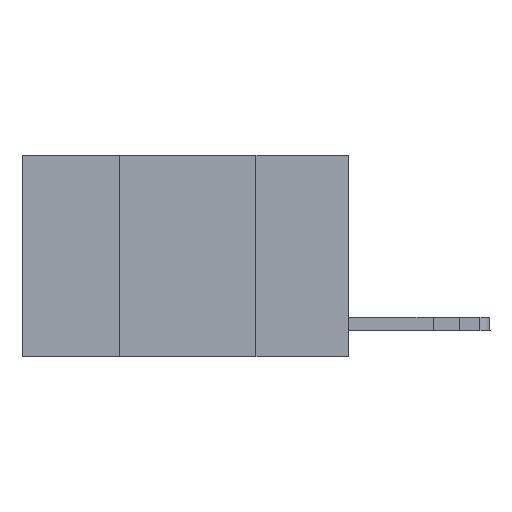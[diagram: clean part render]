
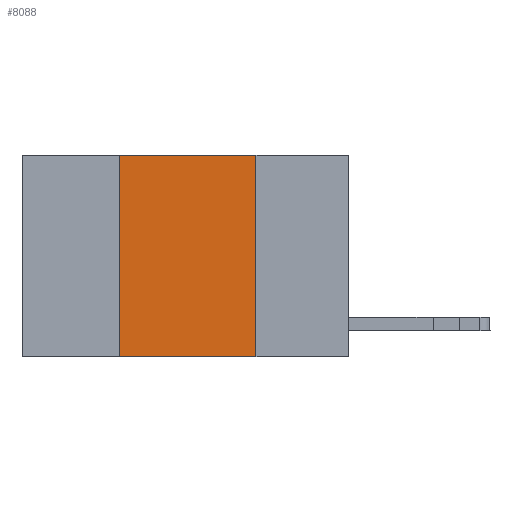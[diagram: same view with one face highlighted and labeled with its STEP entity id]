
A CAD part, left-side view. The second image highlights one B-rep face of the part: STEP entity #8088.
In plain terms, the highlighted planar face has unit normal (-1, 0, 0).
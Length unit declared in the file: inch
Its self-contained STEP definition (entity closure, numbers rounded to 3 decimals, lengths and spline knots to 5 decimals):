
#32 = CARTESIAN_POINT ( 'NONE',  ( 0., 0.17, 0. ) ) ;
#846 = LINE ( 'NONE', #9494, #6445 ) ;
#981 = DIRECTION ( 'NONE',  ( 0., 0., -1. ) ) ;
#1046 = VERTEX_POINT ( 'NONE', #12413 ) ;
#1283 = DIRECTION ( 'NONE',  ( 0., -1., 0. ) ) ;
#1828 = AXIS2_PLACEMENT_3D ( 'NONE', #13999, #7618, #981 ) ;
#1960 = DIRECTION ( 'NONE',  ( 0., 0., 1. ) ) ;
#2311 = ORIENTED_EDGE ( 'NONE', *, *, #13377, .F. ) ;
#2514 = CARTESIAN_POINT ( 'NONE',  ( 0., 0.42, -0.37 ) ) ;
#2594 = LINE ( 'NONE', #4907, #7962 ) ;
#2928 = EDGE_CURVE ( 'NONE', #7114, #14189, #13851, .T. ) ;
#3056 = DIRECTION ( 'NONE',  ( 0., 0., -1. ) ) ;
#3088 = FACE_OUTER_BOUND ( 'NONE', #8971, .T. ) ;
#4907 = CARTESIAN_POINT ( 'NONE',  ( 0., 0.6, -0.37 ) ) ;
#5120 = EDGE_CURVE ( 'NONE', #12855, #1046, #2594, .T. ) ;
#5197 = CARTESIAN_POINT ( 'NONE',  ( 0., 0.17, 0. ) ) ;
#5339 = VECTOR ( 'NONE', #1283, 39.37008 ) ;
#5457 = PLANE ( 'NONE',  #1828 ) ;
#5547 = ORIENTED_EDGE ( 'NONE', *, *, #2928, .F. ) ;
#6210 = ORIENTED_EDGE ( 'NONE', *, *, #5120, .T. ) ;
#6269 = EDGE_CURVE ( 'NONE', #12855, #7114, #846, .T. ) ;
#6445 = VECTOR ( 'NONE', #1960, 39.37008 ) ;
#7114 = VERTEX_POINT ( 'NONE', #8758 ) ;
#7618 = DIRECTION ( 'NONE',  ( 1., 0., 0. ) ) ;
#7826 = LINE ( 'NONE', #5197, #10617 ) ;
#7962 = VECTOR ( 'NONE', #8107, 39.37008 ) ;
#8088 = ADVANCED_FACE ( 'NONE', ( #3088 ), #5457, .F. ) ;
#8107 = DIRECTION ( 'NONE',  ( 0., -1., 0. ) ) ;
#8758 = CARTESIAN_POINT ( 'NONE',  ( 0., 0.42, 0. ) ) ;
#8971 = EDGE_LOOP ( 'NONE', ( #2311, #5547, #11166, #6210 ) ) ;
#9494 = CARTESIAN_POINT ( 'NONE',  ( 0., 0.42, 0. ) ) ;
#10617 = VECTOR ( 'NONE', #3056, 39.37008 ) ;
#11045 = CARTESIAN_POINT ( 'NONE',  ( 0., 0.6, 0. ) ) ;
#11166 = ORIENTED_EDGE ( 'NONE', *, *, #6269, .F. ) ;
#12413 = CARTESIAN_POINT ( 'NONE',  ( 0., 0.17, -0.37 ) ) ;
#12855 = VERTEX_POINT ( 'NONE', #2514 ) ;
#13377 = EDGE_CURVE ( 'NONE', #14189, #1046, #7826, .T. ) ;
#13851 = LINE ( 'NONE', #11045, #5339 ) ;
#13999 = CARTESIAN_POINT ( 'NONE',  ( 0., 0.6, 0. ) ) ;
#14189 = VERTEX_POINT ( 'NONE', #32 ) ;
